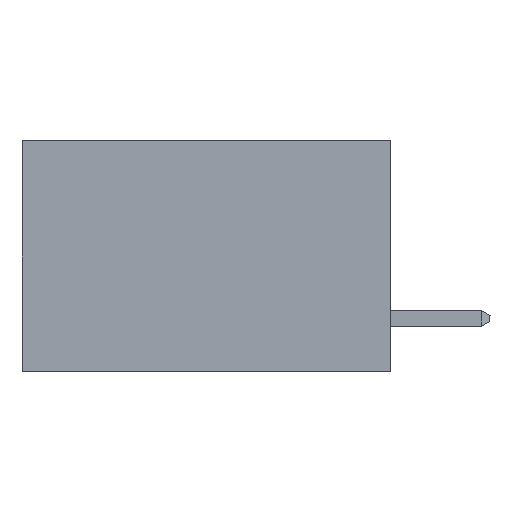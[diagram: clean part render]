
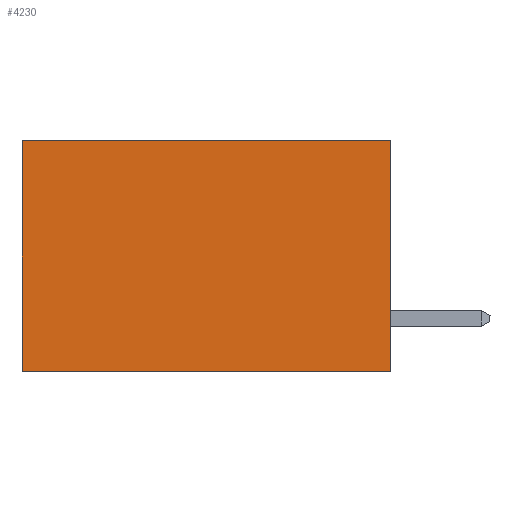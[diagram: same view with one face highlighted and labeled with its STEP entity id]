
A CAD part, left-side view. The second image highlights one B-rep face of the part: STEP entity #4230.
In plain terms, the highlighted planar face has unit normal (-1, 0, 0).
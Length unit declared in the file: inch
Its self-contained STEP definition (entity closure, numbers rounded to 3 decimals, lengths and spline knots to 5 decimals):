
#970 = VECTOR ( 'NONE', #5599, 39.37008 ) ;
#1193 = VECTOR ( 'NONE', #7580, 39.37008 ) ;
#1202 = ORIENTED_EDGE ( 'NONE', *, *, #8025, .T. ) ;
#1214 = VERTEX_POINT ( 'NONE', #7532 ) ;
#1313 = VERTEX_POINT ( 'NONE', #7750 ) ;
#1376 = ORIENTED_EDGE ( 'NONE', *, *, #4394, .F. ) ;
#1696 = VECTOR ( 'NONE', #9823, 39.37008 ) ;
#1703 = VERTEX_POINT ( 'NONE', #8078 ) ;
#1778 = EDGE_LOOP ( 'NONE', ( #1202, #9638, #1376, #8060 ) ) ;
#2059 = DIRECTION ( 'NONE',  ( 0., 0., -1. ) ) ;
#2637 = AXIS2_PLACEMENT_3D ( 'NONE', #6475, #4613, #4440 ) ;
#3067 = LINE ( 'NONE', #6913, #1193 ) ;
#3111 = LINE ( 'NONE', #5346, #970 ) ;
#3476 = EDGE_CURVE ( 'NONE', #1703, #1214, #3067, .T. ) ;
#3865 = FACE_OUTER_BOUND ( 'NONE', #1778, .T. ) ;
#4230 = ADVANCED_FACE ( 'NONE', ( #3865 ), #4658, .F. ) ;
#4394 = EDGE_CURVE ( 'NONE', #1703, #4589, #3111, .T. ) ;
#4440 = DIRECTION ( 'NONE',  ( 0., 0., -1. ) ) ;
#4589 = VERTEX_POINT ( 'NONE', #9687 ) ;
#4613 = DIRECTION ( 'NONE',  ( 1., 0., 0. ) ) ;
#4658 = PLANE ( 'NONE',  #2637 ) ;
#5169 = VECTOR ( 'NONE', #2059, 39.37008 ) ;
#5346 = CARTESIAN_POINT ( 'NONE',  ( 0.277, 0., -0.37 ) ) ;
#5599 = DIRECTION ( 'NONE',  ( 0., 0., -1. ) ) ;
#6162 = CARTESIAN_POINT ( 'NONE',  ( 0.277, 0., -0.37 ) ) ;
#6475 = CARTESIAN_POINT ( 'NONE',  ( 0.277, 0., -0.37 ) ) ;
#6913 = CARTESIAN_POINT ( 'NONE',  ( 0.277, 0., 0. ) ) ;
#7125 = CARTESIAN_POINT ( 'NONE',  ( 0.277, 0.59, -0.37 ) ) ;
#7504 = LINE ( 'NONE', #7125, #5169 ) ;
#7532 = CARTESIAN_POINT ( 'NONE',  ( 0.277, 0.59, 0. ) ) ;
#7580 = DIRECTION ( 'NONE',  ( 0., 1., 0. ) ) ;
#7750 = CARTESIAN_POINT ( 'NONE',  ( 0.277, 0.59, -0.37 ) ) ;
#8025 = EDGE_CURVE ( 'NONE', #1214, #1313, #7504, .T. ) ;
#8060 = ORIENTED_EDGE ( 'NONE', *, *, #3476, .T. ) ;
#8078 = CARTESIAN_POINT ( 'NONE',  ( 0.277, 0., 0. ) ) ;
#8675 = EDGE_CURVE ( 'NONE', #4589, #1313, #9710, .T. ) ;
#9638 = ORIENTED_EDGE ( 'NONE', *, *, #8675, .F. ) ;
#9687 = CARTESIAN_POINT ( 'NONE',  ( 0.277, 0., -0.37 ) ) ;
#9710 = LINE ( 'NONE', #6162, #1696 ) ;
#9823 = DIRECTION ( 'NONE',  ( 0., 1., 0. ) ) ;
